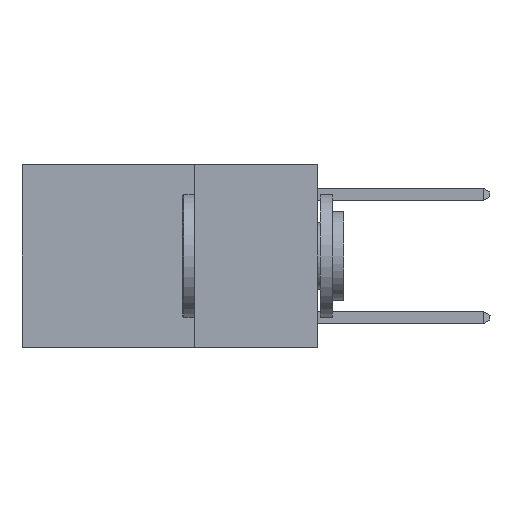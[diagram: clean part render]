
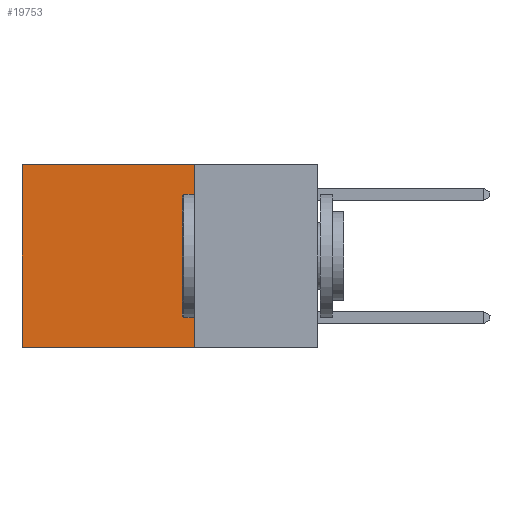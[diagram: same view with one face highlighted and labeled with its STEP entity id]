
A CAD part, left-side view. The second image highlights one B-rep face of the part: STEP entity #19753.
In plain terms, the highlighted planar face has unit normal (-1, 0, 0).
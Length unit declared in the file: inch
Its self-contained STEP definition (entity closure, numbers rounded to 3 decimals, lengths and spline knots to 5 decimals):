
#991 = ORIENTED_EDGE ( 'NONE', *, *, #3814, .T. ) ;
#1006 = FACE_OUTER_BOUND ( 'NONE', #7755, .T. ) ;
#2225 = DIRECTION ( 'NONE',  ( 0., 0., -1. ) ) ;
#2745 = EDGE_CURVE ( 'NONE', #23323, #7379, #30557, .T. ) ;
#3349 = AXIS2_PLACEMENT_3D ( 'NONE', #5241, #9963, #14784 ) ;
#3374 = LINE ( 'NONE', #20624, #28798 ) ;
#3621 = ORIENTED_EDGE ( 'NONE', *, *, #27638, .F. ) ;
#3814 = EDGE_CURVE ( 'NONE', #21303, #11892, #15285, .T. ) ;
#5241 = CARTESIAN_POINT ( 'NONE',  ( 0.2625, 0.25, 0. ) ) ;
#5321 = LINE ( 'NONE', #7020, #25085 ) ;
#6401 = CARTESIAN_POINT ( 'NONE',  ( 0.2625, 0.6, 0. ) ) ;
#7020 = CARTESIAN_POINT ( 'NONE',  ( 0.2625, 0.25, 0. ) ) ;
#7379 = VERTEX_POINT ( 'NONE', #16126 ) ;
#7755 = EDGE_LOOP ( 'NONE', ( #991, #3621, #18999, #15546 ) ) ;
#9599 = CARTESIAN_POINT ( 'NONE',  ( 0.2625, 0.25, 0. ) ) ;
#9963 = DIRECTION ( 'NONE',  ( 1., 0., 0. ) ) ;
#10345 = PLANE ( 'NONE',  #3349 ) ;
#11086 = VECTOR ( 'NONE', #2225, 39.37008 ) ;
#11892 = VERTEX_POINT ( 'NONE', #29761 ) ;
#14784 = DIRECTION ( 'NONE',  ( 0., 0., -1. ) ) ;
#15285 = LINE ( 'NONE', #6401, #26805 ) ;
#15546 = ORIENTED_EDGE ( 'NONE', *, *, #18887, .T. ) ;
#15621 = DIRECTION ( 'NONE',  ( 0., 1., 0. ) ) ;
#16126 = CARTESIAN_POINT ( 'NONE',  ( 0.2625, 0.25, -0.37 ) ) ;
#16238 = CARTESIAN_POINT ( 'NONE',  ( 0.2625, 0.6, 0. ) ) ;
#18887 = EDGE_CURVE ( 'NONE', #23323, #21303, #5321, .T. ) ;
#18999 = ORIENTED_EDGE ( 'NONE', *, *, #2745, .F. ) ;
#19753 = ADVANCED_FACE ( 'NONE', ( #1006 ), #10345, .F. ) ;
#20624 = CARTESIAN_POINT ( 'NONE',  ( 0.2625, 0.25, -0.37 ) ) ;
#21245 = DIRECTION ( 'NONE',  ( 0., 0., -1. ) ) ;
#21303 = VERTEX_POINT ( 'NONE', #16238 ) ;
#23323 = VERTEX_POINT ( 'NONE', #24954 ) ;
#24338 = DIRECTION ( 'NONE',  ( 0., 1., 0. ) ) ;
#24954 = CARTESIAN_POINT ( 'NONE',  ( 0.2625, 0.25, 0. ) ) ;
#25085 = VECTOR ( 'NONE', #24338, 39.37008 ) ;
#26805 = VECTOR ( 'NONE', #21245, 39.37008 ) ;
#27638 = EDGE_CURVE ( 'NONE', #7379, #11892, #3374, .T. ) ;
#28798 = VECTOR ( 'NONE', #15621, 39.37008 ) ;
#29761 = CARTESIAN_POINT ( 'NONE',  ( 0.2625, 0.6, -0.37 ) ) ;
#30557 = LINE ( 'NONE', #9599, #11086 ) ;
